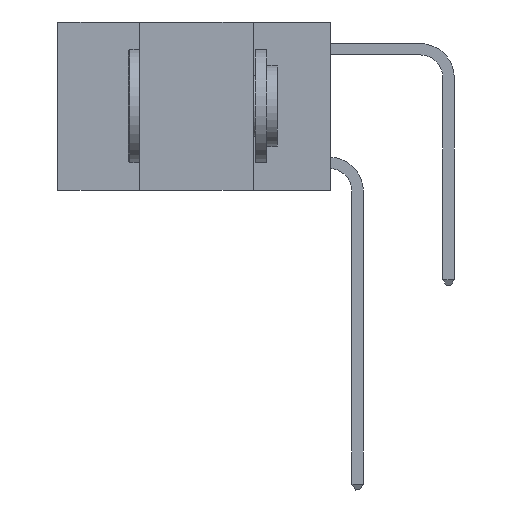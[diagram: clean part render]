
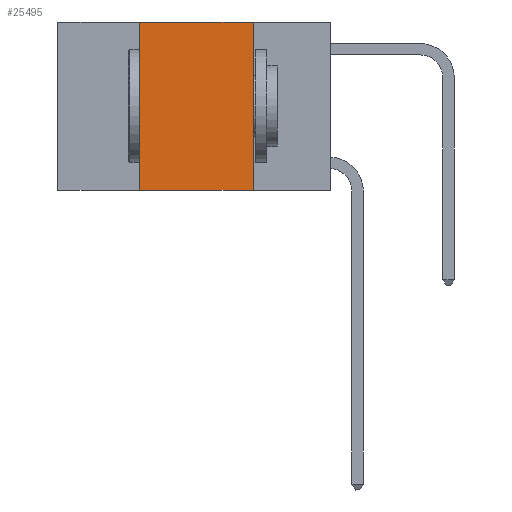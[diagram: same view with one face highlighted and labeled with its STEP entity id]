
A CAD part, left-side view. The second image highlights one B-rep face of the part: STEP entity #25495.
In plain terms, the highlighted planar face has unit normal (-1, 0, 0).
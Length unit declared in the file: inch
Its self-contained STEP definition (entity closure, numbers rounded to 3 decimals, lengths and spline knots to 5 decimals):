
#981 = EDGE_CURVE ( 'NONE', #28261, #8288, #29773, .T. ) ;
#1185 = VECTOR ( 'NONE', #33345, 39.37008 ) ;
#2563 = EDGE_CURVE ( 'NONE', #8288, #10083, #31307, .T. ) ;
#2882 = DIRECTION ( 'NONE',  ( 0., -1., 0. ) ) ;
#3020 = EDGE_CURVE ( 'NONE', #28261, #4709, #25312, .T. ) ;
#3636 = DIRECTION ( 'NONE',  ( 0., 0., -1. ) ) ;
#4709 = VERTEX_POINT ( 'NONE', #14324 ) ;
#5695 = DIRECTION ( 'NONE',  ( 1., 0., 0. ) ) ;
#6501 = DIRECTION ( 'NONE',  ( 0., 0., 1. ) ) ;
#8288 = VERTEX_POINT ( 'NONE', #8958 ) ;
#8958 = CARTESIAN_POINT ( 'NONE',  ( 0., 0.42, 0. ) ) ;
#10083 = VERTEX_POINT ( 'NONE', #14362 ) ;
#11843 = VECTOR ( 'NONE', #6501, 39.37008 ) ;
#12015 = ORIENTED_EDGE ( 'NONE', *, *, #25869, .F. ) ;
#13304 = CARTESIAN_POINT ( 'NONE',  ( 0., 0.6, 0. ) ) ;
#13674 = ORIENTED_EDGE ( 'NONE', *, *, #2563, .F. ) ;
#14324 = CARTESIAN_POINT ( 'NONE',  ( 0., 0.17, -0.37 ) ) ;
#14362 = CARTESIAN_POINT ( 'NONE',  ( 0., 0.17, 0. ) ) ;
#16800 = CARTESIAN_POINT ( 'NONE',  ( 0., 0.42, -0.37 ) ) ;
#19923 = CARTESIAN_POINT ( 'NONE',  ( 0., 0.17, 0. ) ) ;
#21462 = VECTOR ( 'NONE', #2882, 39.37008 ) ;
#22805 = DIRECTION ( 'NONE',  ( 0., 0., -1. ) ) ;
#24190 = CARTESIAN_POINT ( 'NONE',  ( 0., 0.6, 0. ) ) ;
#24683 = LINE ( 'NONE', #19923, #29538 ) ;
#25312 = LINE ( 'NONE', #26151, #21462 ) ;
#25495 = ADVANCED_FACE ( 'NONE', ( #26240 ), #26902, .F. ) ;
#25869 = EDGE_CURVE ( 'NONE', #10083, #4709, #24683, .T. ) ;
#26151 = CARTESIAN_POINT ( 'NONE',  ( 0., 0.6, -0.37 ) ) ;
#26240 = FACE_OUTER_BOUND ( 'NONE', #33532, .T. ) ;
#26902 = PLANE ( 'NONE',  #27375 ) ;
#27375 = AXIS2_PLACEMENT_3D ( 'NONE', #24190, #5695, #3636 ) ;
#27555 = CARTESIAN_POINT ( 'NONE',  ( 0., 0.42, 0. ) ) ;
#28261 = VERTEX_POINT ( 'NONE', #16800 ) ;
#29538 = VECTOR ( 'NONE', #22805, 39.37008 ) ;
#29773 = LINE ( 'NONE', #27555, #11843 ) ;
#31307 = LINE ( 'NONE', #13304, #1185 ) ;
#31715 = ORIENTED_EDGE ( 'NONE', *, *, #981, .F. ) ;
#31870 = ORIENTED_EDGE ( 'NONE', *, *, #3020, .T. ) ;
#33345 = DIRECTION ( 'NONE',  ( 0., -1., 0. ) ) ;
#33532 = EDGE_LOOP ( 'NONE', ( #12015, #13674, #31715, #31870 ) ) ;
